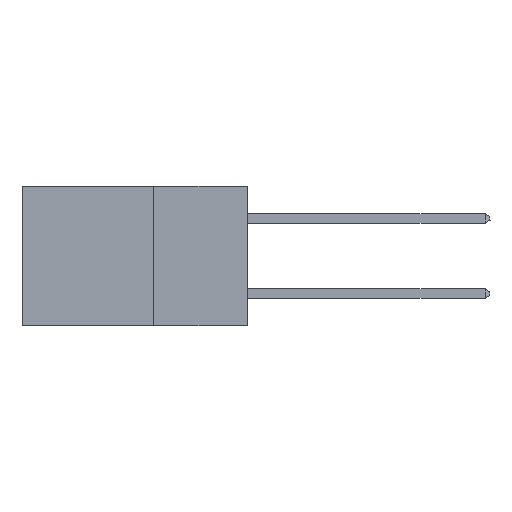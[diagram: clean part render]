
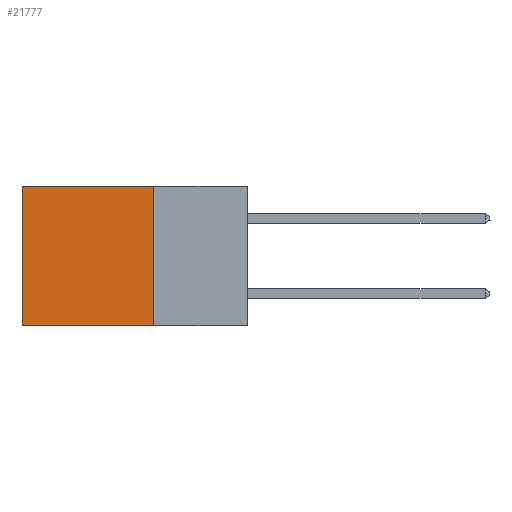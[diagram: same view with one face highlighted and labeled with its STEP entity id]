
A CAD part, left-side view. The second image highlights one B-rep face of the part: STEP entity #21777.
In plain terms, the highlighted planar face has unit normal (-1, 0, 0).
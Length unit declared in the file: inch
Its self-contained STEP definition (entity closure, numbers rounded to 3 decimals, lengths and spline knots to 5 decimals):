
#574 = CARTESIAN_POINT ( 'NONE',  ( 0.298, 0.25, -0.37 ) ) ;
#2410 = FACE_OUTER_BOUND ( 'NONE', #28724, .T. ) ;
#3478 = EDGE_CURVE ( 'NONE', #16455, #6055, #26382, .T. ) ;
#6055 = VERTEX_POINT ( 'NONE', #17864 ) ;
#6230 = VECTOR ( 'NONE', #15403, 39.37008 ) ;
#6653 = VERTEX_POINT ( 'NONE', #12129 ) ;
#7584 = DIRECTION ( 'NONE',  ( 0., 1., 0. ) ) ;
#7928 = DIRECTION ( 'NONE',  ( 1., 0., 0. ) ) ;
#8323 = EDGE_CURVE ( 'NONE', #21486, #6653, #20742, .T. ) ;
#9857 = EDGE_CURVE ( 'NONE', #6653, #6055, #27720, .T. ) ;
#9982 = LINE ( 'NONE', #27718, #27293 ) ;
#10379 = CARTESIAN_POINT ( 'NONE',  ( 0.298, 0.25, 0. ) ) ;
#12129 = CARTESIAN_POINT ( 'NONE',  ( 0.298, 0.6, 0. ) ) ;
#12238 = ORIENTED_EDGE ( 'NONE', *, *, #16962, .F. ) ;
#12241 = DIRECTION ( 'NONE',  ( 0., 0., -1. ) ) ;
#14475 = ORIENTED_EDGE ( 'NONE', *, *, #8323, .T. ) ;
#14612 = CARTESIAN_POINT ( 'NONE',  ( 0.298, 0.6, 0. ) ) ;
#15059 = VECTOR ( 'NONE', #7584, 39.37008 ) ;
#15403 = DIRECTION ( 'NONE',  ( 0., 1., 0. ) ) ;
#15761 = PLANE ( 'NONE',  #22108 ) ;
#16455 = VERTEX_POINT ( 'NONE', #574 ) ;
#16962 = EDGE_CURVE ( 'NONE', #21486, #16455, #9982, .T. ) ;
#17831 = DIRECTION ( 'NONE',  ( 0., 0., -1. ) ) ;
#17864 = CARTESIAN_POINT ( 'NONE',  ( 0.298, 0.6, -0.37 ) ) ;
#20742 = LINE ( 'NONE', #22313, #6230 ) ;
#21486 = VERTEX_POINT ( 'NONE', #31975 ) ;
#21777 = ADVANCED_FACE ( 'NONE', ( #2410 ), #15761, .F. ) ;
#22108 = AXIS2_PLACEMENT_3D ( 'NONE', #10379, #7928, #28003 ) ;
#22313 = CARTESIAN_POINT ( 'NONE',  ( 0.298, 0.25, 0. ) ) ;
#22623 = CARTESIAN_POINT ( 'NONE',  ( 0.298, 0.25, -0.37 ) ) ;
#24274 = ORIENTED_EDGE ( 'NONE', *, *, #9857, .T. ) ;
#25786 = ORIENTED_EDGE ( 'NONE', *, *, #3478, .F. ) ;
#26382 = LINE ( 'NONE', #22623, #15059 ) ;
#27293 = VECTOR ( 'NONE', #17831, 39.37008 ) ;
#27718 = CARTESIAN_POINT ( 'NONE',  ( 0.298, 0.25, 0. ) ) ;
#27720 = LINE ( 'NONE', #14612, #31219 ) ;
#28003 = DIRECTION ( 'NONE',  ( 0., 0., -1. ) ) ;
#28724 = EDGE_LOOP ( 'NONE', ( #24274, #25786, #12238, #14475 ) ) ;
#31219 = VECTOR ( 'NONE', #12241, 39.37008 ) ;
#31975 = CARTESIAN_POINT ( 'NONE',  ( 0.298, 0.25, 0. ) ) ;
